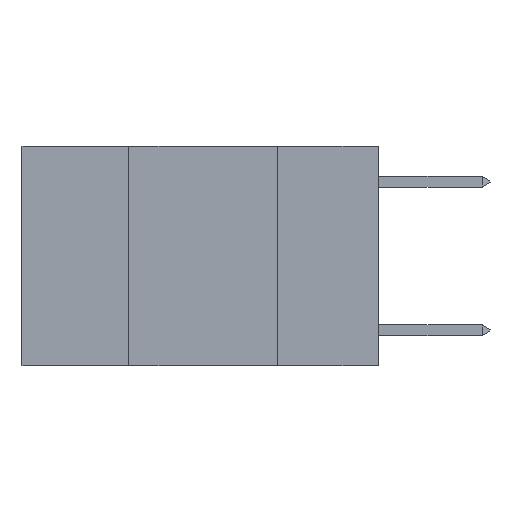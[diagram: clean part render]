
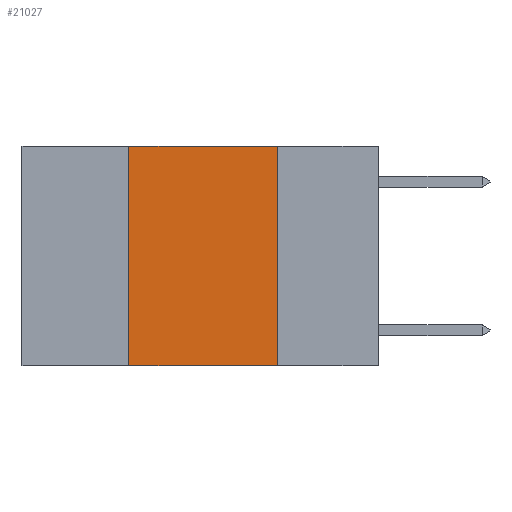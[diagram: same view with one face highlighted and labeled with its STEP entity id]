
A CAD part, left-side view. The second image highlights one B-rep face of the part: STEP entity #21027.
In plain terms, the highlighted planar face has unit normal (-1, 0, 0).
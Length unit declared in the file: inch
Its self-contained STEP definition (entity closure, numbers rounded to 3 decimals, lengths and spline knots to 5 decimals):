
#1292 = LINE ( 'NONE', #3690, #3266 ) ;
#3226 = DIRECTION ( 'NONE',  ( 0., 0., -1. ) ) ;
#3266 = VECTOR ( 'NONE', #3226, 39.37008 ) ;
#3566 = CARTESIAN_POINT ( 'NONE',  ( 0., 0.42, 0. ) ) ;
#3690 = CARTESIAN_POINT ( 'NONE',  ( 0., 0.17, 0. ) ) ;
#3892 = EDGE_CURVE ( 'NONE', #24216, #13485, #27997, .T. ) ;
#4211 = CARTESIAN_POINT ( 'NONE',  ( 0., 0.17, -0.37 ) ) ;
#4344 = PLANE ( 'NONE',  #22502 ) ;
#5976 = VECTOR ( 'NONE', #28476, 39.37008 ) ;
#6710 = VERTEX_POINT ( 'NONE', #4211 ) ;
#9999 = EDGE_CURVE ( 'NONE', #17317, #6710, #1292, .T. ) ;
#13073 = CARTESIAN_POINT ( 'NONE',  ( 0., 0.42, -0.37 ) ) ;
#13485 = VERTEX_POINT ( 'NONE', #16924 ) ;
#13536 = VECTOR ( 'NONE', #17742, 39.37008 ) ;
#14187 = CARTESIAN_POINT ( 'NONE',  ( 0., 0.6, -0.37 ) ) ;
#14492 = DIRECTION ( 'NONE',  ( 0., 0., -1. ) ) ;
#16742 = CARTESIAN_POINT ( 'NONE',  ( 0., 0.6, 0. ) ) ;
#16924 = CARTESIAN_POINT ( 'NONE',  ( 0., 0.42, 0. ) ) ;
#17317 = VERTEX_POINT ( 'NONE', #27707 ) ;
#17449 = ORIENTED_EDGE ( 'NONE', *, *, #3892, .F. ) ;
#17742 = DIRECTION ( 'NONE',  ( 0., 0., 1. ) ) ;
#17921 = CARTESIAN_POINT ( 'NONE',  ( 0., 0.6, 0. ) ) ;
#18167 = EDGE_LOOP ( 'NONE', ( #29361, #27352, #17449, #30113 ) ) ;
#18390 = LINE ( 'NONE', #17921, #24133 ) ;
#18680 = LINE ( 'NONE', #14187, #5976 ) ;
#19146 = EDGE_CURVE ( 'NONE', #24216, #6710, #18680, .T. ) ;
#21027 = ADVANCED_FACE ( 'NONE', ( #26524 ), #4344, .F. ) ;
#22502 = AXIS2_PLACEMENT_3D ( 'NONE', #16742, #24116, #14492 ) ;
#23370 = DIRECTION ( 'NONE',  ( 0., -1., 0. ) ) ;
#24116 = DIRECTION ( 'NONE',  ( 1., 0., 0. ) ) ;
#24133 = VECTOR ( 'NONE', #23370, 39.37008 ) ;
#24216 = VERTEX_POINT ( 'NONE', #13073 ) ;
#25100 = EDGE_CURVE ( 'NONE', #13485, #17317, #18390, .T. ) ;
#26524 = FACE_OUTER_BOUND ( 'NONE', #18167, .T. ) ;
#27352 = ORIENTED_EDGE ( 'NONE', *, *, #25100, .F. ) ;
#27707 = CARTESIAN_POINT ( 'NONE',  ( 0., 0.17, 0. ) ) ;
#27997 = LINE ( 'NONE', #3566, #13536 ) ;
#28476 = DIRECTION ( 'NONE',  ( 0., -1., 0. ) ) ;
#29361 = ORIENTED_EDGE ( 'NONE', *, *, #9999, .F. ) ;
#30113 = ORIENTED_EDGE ( 'NONE', *, *, #19146, .T. ) ;
